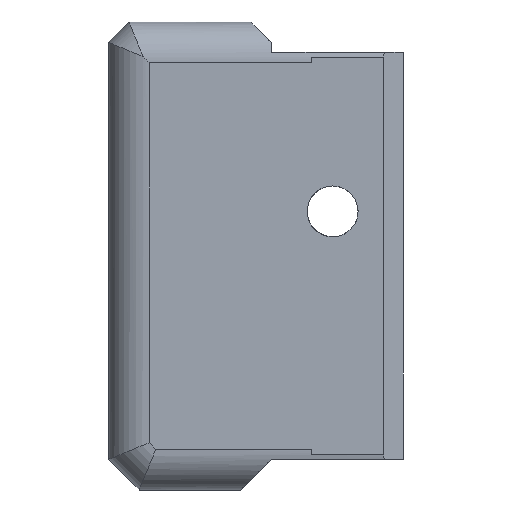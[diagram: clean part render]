
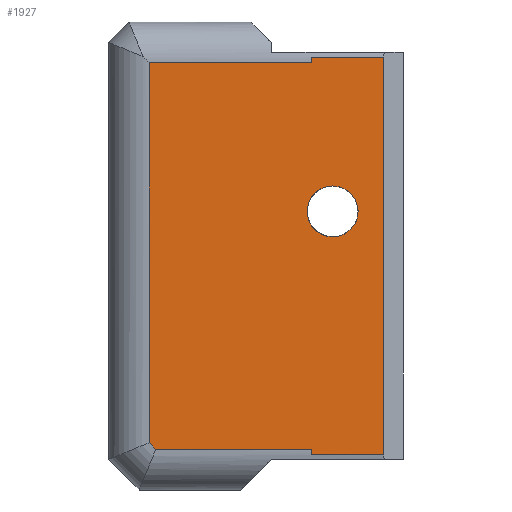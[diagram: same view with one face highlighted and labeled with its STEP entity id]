
A CAD part, left-side view. The second image highlights one B-rep face of the part: STEP entity #1927.
In plain terms, the highlighted planar face has unit normal (-1, 0, 0).
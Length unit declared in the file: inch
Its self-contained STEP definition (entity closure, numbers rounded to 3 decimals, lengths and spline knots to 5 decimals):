
#19=FACE_BOUND('',#240,.T.);
#28=CIRCLE('',#2003,0.09843);
#29=CIRCLE('',#2004,0.09843);
#30=CIRCLE('',#2005,0.09843);
#140=FACE_OUTER_BOUND('',#239,.T.);
#239=EDGE_LOOP('',(#1630,#1631,#1632,#1633,#1634,#1635,#1636,#1637,#1638));
#240=EDGE_LOOP('',(#1639,#1640,#1641));
#406=LINE('',#3046,#622);
#413=LINE('',#3063,#629);
#418=LINE('',#3080,#634);
#446=LINE('',#3182,#662);
#447=LINE('',#3185,#663);
#449=LINE('',#3188,#665);
#450=LINE('',#3190,#666);
#492=LINE('',#3285,#708);
#493=LINE('',#3286,#709);
#622=VECTOR('',#2331,0.3937);
#629=VECTOR('',#2346,0.3937);
#634=VECTOR('',#2363,0.3937);
#662=VECTOR('',#2423,0.3937);
#663=VECTOR('',#2426,0.3937);
#665=VECTOR('',#2430,0.3937);
#666=VECTOR('',#2433,0.3937);
#708=VECTOR('',#2533,0.3937);
#709=VECTOR('',#2534,0.3937);
#814=VERTEX_POINT('',#2915);
#815=VERTEX_POINT('',#2917);
#816=VERTEX_POINT('',#2919);
#835=VERTEX_POINT('',#3032);
#841=VERTEX_POINT('',#3044);
#846=VERTEX_POINT('',#3060);
#847=VERTEX_POINT('',#3062);
#852=VERTEX_POINT('',#3077);
#853=VERTEX_POINT('',#3079);
#877=VERTEX_POINT('',#3180);
#878=VERTEX_POINT('',#3184);
#898=VERTEX_POINT('',#3284);
#1019=EDGE_CURVE('',#815,#814,#28,.T.);
#1020=EDGE_CURVE('',#816,#815,#29,.T.);
#1021=EDGE_CURVE('',#814,#816,#30,.T.);
#1057=EDGE_CURVE('',#841,#835,#406,.T.);
#1065=EDGE_CURVE('',#846,#847,#413,.T.);
#1074=EDGE_CURVE('',#852,#853,#418,.T.);
#1109=EDGE_CURVE('',#841,#877,#446,.T.);
#1110=EDGE_CURVE('',#878,#853,#447,.T.);
#1112=EDGE_CURVE('',#877,#847,#449,.T.);
#1113=EDGE_CURVE('',#846,#878,#450,.T.);
#1158=EDGE_CURVE('',#898,#852,#492,.T.);
#1159=EDGE_CURVE('',#835,#898,#493,.T.);
#1630=ORIENTED_EDGE('',*,*,#1065,.F.);
#1631=ORIENTED_EDGE('',*,*,#1113,.T.);
#1632=ORIENTED_EDGE('',*,*,#1110,.T.);
#1633=ORIENTED_EDGE('',*,*,#1074,.F.);
#1634=ORIENTED_EDGE('',*,*,#1158,.F.);
#1635=ORIENTED_EDGE('',*,*,#1159,.F.);
#1636=ORIENTED_EDGE('',*,*,#1057,.F.);
#1637=ORIENTED_EDGE('',*,*,#1109,.T.);
#1638=ORIENTED_EDGE('',*,*,#1112,.T.);
#1639=ORIENTED_EDGE('',*,*,#1019,.T.);
#1640=ORIENTED_EDGE('',*,*,#1021,.T.);
#1641=ORIENTED_EDGE('',*,*,#1020,.T.);
#1840=PLANE('',#2077);
#1927=ADVANCED_FACE('',(#140,#19),#1840,.T.);
#2003=AXIS2_PLACEMENT_3D('',#2918,#2272,#2273);
#2004=AXIS2_PLACEMENT_3D('',#2920,#2274,#2275);
#2005=AXIS2_PLACEMENT_3D('',#2921,#2276,#2277);
#2077=AXIS2_PLACEMENT_3D('',#3283,#2531,#2532);
#2272=DIRECTION('center_axis',(1.,0.,0.));
#2273=DIRECTION('ref_axis',(0.,0.,-1.));
#2274=DIRECTION('center_axis',(1.,0.,0.));
#2275=DIRECTION('ref_axis',(0.,0.,-1.));
#2276=DIRECTION('center_axis',(1.,0.,0.));
#2277=DIRECTION('ref_axis',(0.,0.,-1.));
#2331=DIRECTION('',(0.,1.,0.));
#2346=DIRECTION('',(0.,0.,-1.));
#2363=DIRECTION('',(0.,-1.,0.));
#2423=DIRECTION('',(0.,0.,-1.));
#2426=DIRECTION('',(0.,0.,-1.));
#2430=DIRECTION('',(0.,-1.,0.));
#2433=DIRECTION('',(0.,1.,0.));
#2531=DIRECTION('center_axis',(-1.,0.,0.));
#2532=DIRECTION('ref_axis',(0.,0.,-1.));
#2533=DIRECTION('',(0.,0.,1.));
#2534=DIRECTION('',(0.,0.707,0.707));
#2915=CARTESIAN_POINT('',(-0.59478,2.8771,-1.24988));
#2917=CARTESIAN_POINT('',(-0.59478,2.95733,-1.29128));
#2918=CARTESIAN_POINT('Origin',(-0.59478,2.8771,-1.34831));
#2919=CARTESIAN_POINT('',(-0.59478,2.95733,-1.40533));
#2920=CARTESIAN_POINT('Origin',(-0.59478,2.8771,-1.34831));
#2921=CARTESIAN_POINT('Origin',(-0.59478,2.8771,-1.34831));
#3032=CARTESIAN_POINT('',(-0.59478,3.56101,-2.26882));
#3044=CARTESIAN_POINT('',(-0.59478,2.95733,-2.26882));
#3046=CARTESIAN_POINT('',(-0.59478,3.74435,-2.26882));
#3060=CARTESIAN_POINT('',(-0.59478,2.68174,-0.75083));
#3062=CARTESIAN_POINT('',(-0.59478,2.68176,-2.29076));
#3063=CARTESIAN_POINT('',(-0.59478,2.68175,-1.46121));
#3077=CARTESIAN_POINT('',(-0.59478,3.58687,-0.77276));
#3079=CARTESIAN_POINT('',(-0.59478,2.95733,-0.77276));
#3080=CARTESIAN_POINT('',(-0.59478,3.74435,-0.77276));
#3180=CARTESIAN_POINT('',(-0.59478,2.95733,-2.29076));
#3182=CARTESIAN_POINT('',(-0.59478,2.95733,-0.72977));
#3184=CARTESIAN_POINT('',(-0.59478,2.95733,-0.75083));
#3185=CARTESIAN_POINT('',(-0.59478,2.95733,-0.72977));
#3188=CARTESIAN_POINT('',(-0.59478,3.74435,-2.29076));
#3190=CARTESIAN_POINT('',(-0.59478,3.74435,-0.75083));
#3283=CARTESIAN_POINT('Origin',(-0.59478,3.74435,-0.61528));
#3284=CARTESIAN_POINT('',(-0.59478,3.58687,-2.24296));
#3285=CARTESIAN_POINT('',(-0.59478,3.58687,-1.06804));
#3286=CARTESIAN_POINT('',(-0.59478,4.02669,-1.80314));
